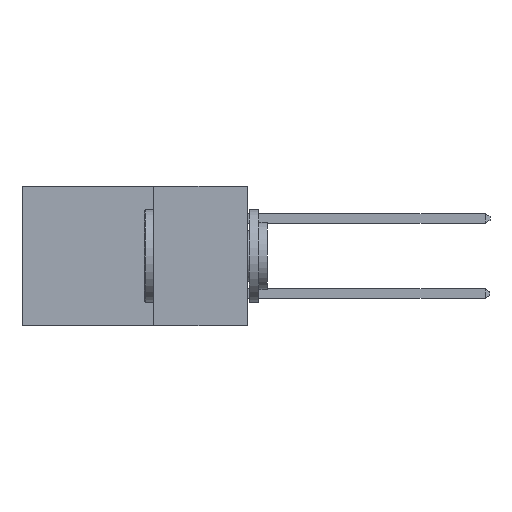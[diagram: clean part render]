
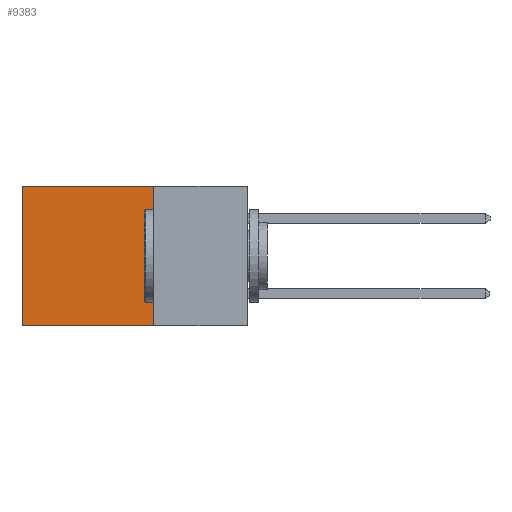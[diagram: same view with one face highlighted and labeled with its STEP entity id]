
A CAD part, left-side view. The second image highlights one B-rep face of the part: STEP entity #9383.
In plain terms, the highlighted planar face has unit normal (-1, 0, 0).
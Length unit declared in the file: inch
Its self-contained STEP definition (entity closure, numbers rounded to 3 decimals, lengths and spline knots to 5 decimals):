
#49 = DIRECTION ( 'NONE',  ( 0., 0., -1. ) ) ;
#475 = CARTESIAN_POINT ( 'NONE',  ( 0.298, 0.25, -0.37 ) ) ;
#559 = CARTESIAN_POINT ( 'NONE',  ( 0.298, 0.6, 0. ) ) ;
#620 = LINE ( 'NONE', #20018, #5571 ) ;
#2028 = DIRECTION ( 'NONE',  ( 0., 0., -1. ) ) ;
#2274 = ORIENTED_EDGE ( 'NONE', *, *, #11082, .F. ) ;
#2777 = FACE_OUTER_BOUND ( 'NONE', #8798, .T. ) ;
#3899 = VECTOR ( 'NONE', #10718, 39.37008 ) ;
#4287 = VERTEX_POINT ( 'NONE', #475 ) ;
#4555 = DIRECTION ( 'NONE',  ( 0., 1., 0. ) ) ;
#4741 = ORIENTED_EDGE ( 'NONE', *, *, #8783, .T. ) ;
#5470 = AXIS2_PLACEMENT_3D ( 'NONE', #6678, #9729, #49 ) ;
#5571 = VECTOR ( 'NONE', #10864, 39.37008 ) ;
#6386 = LINE ( 'NONE', #8417, #17691 ) ;
#6678 = CARTESIAN_POINT ( 'NONE',  ( 0.298, 0.25, 0. ) ) ;
#8270 = VERTEX_POINT ( 'NONE', #559 ) ;
#8417 = CARTESIAN_POINT ( 'NONE',  ( 0.298, 0.6, 0. ) ) ;
#8783 = EDGE_CURVE ( 'NONE', #8270, #17069, #6386, .T. ) ;
#8798 = EDGE_LOOP ( 'NONE', ( #4741, #11341, #2274, #8923 ) ) ;
#8895 = VERTEX_POINT ( 'NONE', #14889 ) ;
#8923 = ORIENTED_EDGE ( 'NONE', *, *, #12390, .T. ) ;
#9163 = CARTESIAN_POINT ( 'NONE',  ( 0.298, 0.25, 0. ) ) ;
#9383 = ADVANCED_FACE ( 'NONE', ( #2777 ), #18901, .F. ) ;
#9729 = DIRECTION ( 'NONE',  ( 1., 0., 0. ) ) ;
#9886 = EDGE_CURVE ( 'NONE', #4287, #17069, #620, .T. ) ;
#10718 = DIRECTION ( 'NONE',  ( 0., 0., -1. ) ) ;
#10864 = DIRECTION ( 'NONE',  ( 0., 1., 0. ) ) ;
#10946 = CARTESIAN_POINT ( 'NONE',  ( 0.298, 0.6, -0.37 ) ) ;
#11082 = EDGE_CURVE ( 'NONE', #8895, #4287, #16322, .T. ) ;
#11341 = ORIENTED_EDGE ( 'NONE', *, *, #9886, .F. ) ;
#12390 = EDGE_CURVE ( 'NONE', #8895, #8270, #19747, .T. ) ;
#13818 = CARTESIAN_POINT ( 'NONE',  ( 0.298, 0.25, 0. ) ) ;
#14889 = CARTESIAN_POINT ( 'NONE',  ( 0.298, 0.25, 0. ) ) ;
#15298 = VECTOR ( 'NONE', #4555, 39.37008 ) ;
#16322 = LINE ( 'NONE', #9163, #3899 ) ;
#17069 = VERTEX_POINT ( 'NONE', #10946 ) ;
#17691 = VECTOR ( 'NONE', #2028, 39.37008 ) ;
#18901 = PLANE ( 'NONE',  #5470 ) ;
#19747 = LINE ( 'NONE', #13818, #15298 ) ;
#20018 = CARTESIAN_POINT ( 'NONE',  ( 0.298, 0.25, -0.37 ) ) ;
